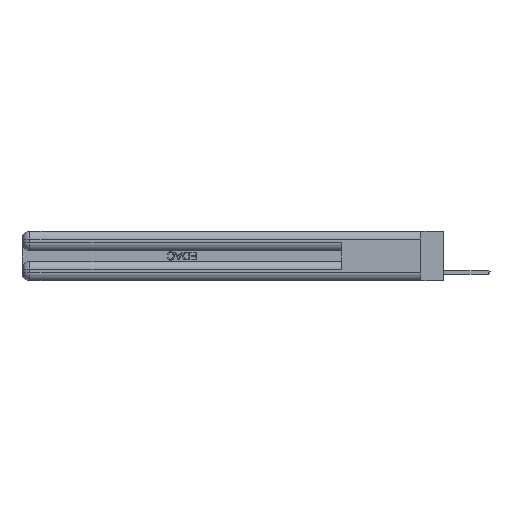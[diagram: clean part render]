
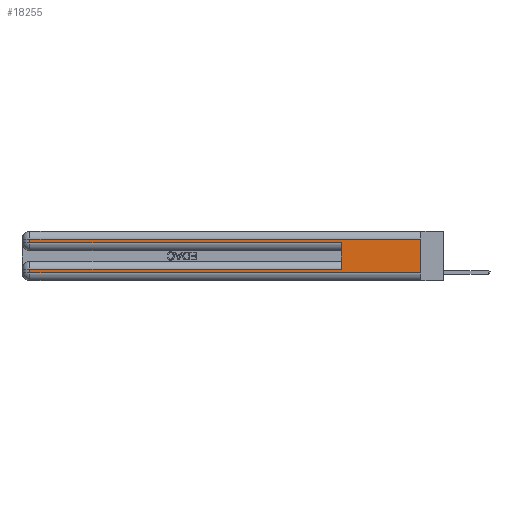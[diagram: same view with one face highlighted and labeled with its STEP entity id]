
A CAD part, left-side view. The second image highlights one B-rep face of the part: STEP entity #18255.
In plain terms, the highlighted planar face has unit normal (-1, 0, 0).
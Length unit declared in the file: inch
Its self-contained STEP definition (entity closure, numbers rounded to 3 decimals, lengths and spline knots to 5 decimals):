
#222 = CARTESIAN_POINT ( 'NONE',  ( 0., 2.94, 0.37 ) ) ;
#349 = ORIENTED_EDGE ( 'NONE', *, *, #33923, .T. ) ;
#2299 = CARTESIAN_POINT ( 'NONE',  ( 0., 0., 0.085 ) ) ;
#2377 = CARTESIAN_POINT ( 'NONE',  ( 0., 0., 0.37 ) ) ;
#2935 = VERTEX_POINT ( 'NONE', #15485 ) ;
#3724 = DIRECTION ( 'NONE',  ( 0., 0., -1. ) ) ;
#4738 = CARTESIAN_POINT ( 'NONE',  ( 0., 0., 0.285 ) ) ;
#4824 = EDGE_CURVE ( 'NONE', #15919, #32992, #10326, .T. ) ;
#5167 = CARTESIAN_POINT ( 'NONE',  ( 0., 0., 0.31 ) ) ;
#5557 = VECTOR ( 'NONE', #19449, 39.37008 ) ;
#6404 = CARTESIAN_POINT ( 'NONE',  ( 0., 2.94, 0.06 ) ) ;
#6551 = VERTEX_POINT ( 'NONE', #8174 ) ;
#7744 = VECTOR ( 'NONE', #27123, 39.37008 ) ;
#8061 = DIRECTION ( 'NONE',  ( 0., 0., 1. ) ) ;
#8174 = CARTESIAN_POINT ( 'NONE',  ( 0., 0., 0.31 ) ) ;
#8249 = EDGE_CURVE ( 'NONE', #6551, #29962, #24491, .T. ) ;
#10010 = VERTEX_POINT ( 'NONE', #24476 ) ;
#10326 = LINE ( 'NONE', #21092, #18658 ) ;
#12530 = EDGE_CURVE ( 'NONE', #6551, #10010, #14150, .T. ) ;
#12691 = VECTOR ( 'NONE', #19632, 39.37008 ) ;
#12902 = DIRECTION ( 'NONE',  ( 0., 0., -1. ) ) ;
#14150 = LINE ( 'NONE', #27508, #5557 ) ;
#15485 = CARTESIAN_POINT ( 'NONE',  ( 0., 2.94, 0.085 ) ) ;
#15919 = VERTEX_POINT ( 'NONE', #32063 ) ;
#16023 = VECTOR ( 'NONE', #12902, 39.37008 ) ;
#17411 = DIRECTION ( 'NONE',  ( 0., -1., 0. ) ) ;
#18143 = LINE ( 'NONE', #2299, #32736 ) ;
#18255 = ADVANCED_FACE ( 'NONE', ( #26447 ), #26796, .F. ) ;
#18301 = ORIENTED_EDGE ( 'NONE', *, *, #12530, .F. ) ;
#18658 = VECTOR ( 'NONE', #8061, 39.37008 ) ;
#19115 = CARTESIAN_POINT ( 'NONE',  ( 0., 0., 0.06 ) ) ;
#19449 = DIRECTION ( 'NONE',  ( 0., 0., -1. ) ) ;
#19632 = DIRECTION ( 'NONE',  ( 0., -1., 0. ) ) ;
#20088 = EDGE_CURVE ( 'NONE', #2935, #27698, #24308, .T. ) ;
#20417 = EDGE_CURVE ( 'NONE', #15919, #2935, #18143, .T. ) ;
#21092 = CARTESIAN_POINT ( 'NONE',  ( 0., 0.6, 0.145 ) ) ;
#21296 = DIRECTION ( 'NONE',  ( 0., 1., 0. ) ) ;
#21613 = CARTESIAN_POINT ( 'NONE',  ( 0., 0.6, 0.285 ) ) ;
#21623 = ORIENTED_EDGE ( 'NONE', *, *, #20417, .T. ) ;
#23345 = VECTOR ( 'NONE', #17411, 39.37008 ) ;
#23715 = LINE ( 'NONE', #4738, #23345 ) ;
#24155 = CARTESIAN_POINT ( 'NONE',  ( 0., 2.94, 0.31 ) ) ;
#24308 = LINE ( 'NONE', #222, #32131 ) ;
#24476 = CARTESIAN_POINT ( 'NONE',  ( 0., 0., 0.06 ) ) ;
#24491 = LINE ( 'NONE', #5167, #7744 ) ;
#24582 = VERTEX_POINT ( 'NONE', #33837 ) ;
#25947 = AXIS2_PLACEMENT_3D ( 'NONE', #2377, #31557, #34375 ) ;
#26261 = CARTESIAN_POINT ( 'NONE',  ( 0., 2.94, 0.37 ) ) ;
#26447 = FACE_OUTER_BOUND ( 'NONE', #31650, .T. ) ;
#26621 = LINE ( 'NONE', #26261, #16023 ) ;
#26679 = ORIENTED_EDGE ( 'NONE', *, *, #8249, .T. ) ;
#26796 = PLANE ( 'NONE',  #25947 ) ;
#27123 = DIRECTION ( 'NONE',  ( 0., 1., 0. ) ) ;
#27508 = CARTESIAN_POINT ( 'NONE',  ( 0., 0., 0.37 ) ) ;
#27698 = VERTEX_POINT ( 'NONE', #6404 ) ;
#28962 = ORIENTED_EDGE ( 'NONE', *, *, #34451, .T. ) ;
#29652 = ORIENTED_EDGE ( 'NONE', *, *, #4824, .F. ) ;
#29962 = VERTEX_POINT ( 'NONE', #24155 ) ;
#31146 = EDGE_CURVE ( 'NONE', #29962, #24582, #26621, .T. ) ;
#31557 = DIRECTION ( 'NONE',  ( 1., 0., 0. ) ) ;
#31650 = EDGE_LOOP ( 'NONE', ( #18301, #26679, #33938, #349, #29652, #21623, #32426, #28962 ) ) ;
#32063 = CARTESIAN_POINT ( 'NONE',  ( 0., 0.6, 0.085 ) ) ;
#32131 = VECTOR ( 'NONE', #3724, 39.37008 ) ;
#32426 = ORIENTED_EDGE ( 'NONE', *, *, #20088, .T. ) ;
#32454 = LINE ( 'NONE', #19115, #12691 ) ;
#32736 = VECTOR ( 'NONE', #21296, 39.37008 ) ;
#32992 = VERTEX_POINT ( 'NONE', #21613 ) ;
#33837 = CARTESIAN_POINT ( 'NONE',  ( 0., 2.94, 0.285 ) ) ;
#33923 = EDGE_CURVE ( 'NONE', #24582, #32992, #23715, .T. ) ;
#33938 = ORIENTED_EDGE ( 'NONE', *, *, #31146, .T. ) ;
#34375 = DIRECTION ( 'NONE',  ( 0., 0., -1. ) ) ;
#34451 = EDGE_CURVE ( 'NONE', #27698, #10010, #32454, .T. ) ;
